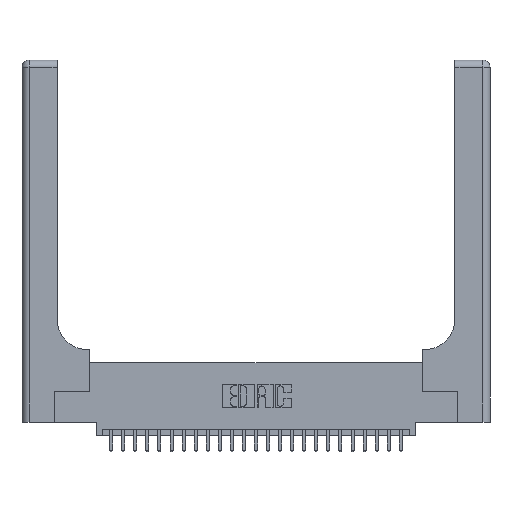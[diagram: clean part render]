
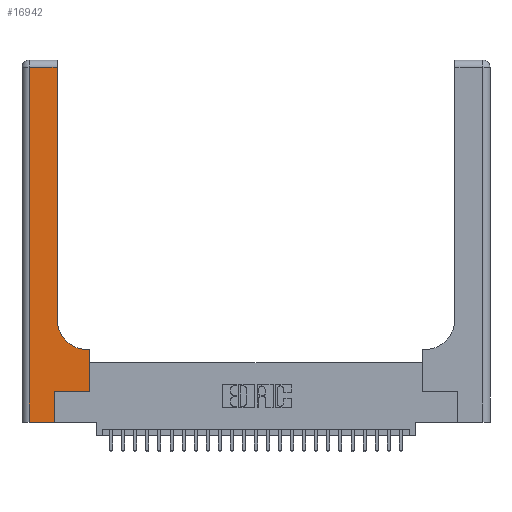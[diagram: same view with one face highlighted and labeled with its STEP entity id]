
A CAD part, top view. The second image highlights one B-rep face of the part: STEP entity #16942.
In plain terms, the highlighted planar face has unit normal (0, 0, 1).
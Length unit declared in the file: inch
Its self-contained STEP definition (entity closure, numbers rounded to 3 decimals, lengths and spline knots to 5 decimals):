
#304 = LINE ( 'NONE', #21245, #10974 ) ;
#325 = FACE_OUTER_BOUND ( 'NONE', #7812, .T. ) ;
#400 = DIRECTION ( 'NONE',  ( 1., 0., 0. ) ) ;
#538 = CARTESIAN_POINT ( 'NONE',  ( 0.269, 0., 0.37 ) ) ;
#1228 = VERTEX_POINT ( 'NONE', #18235 ) ;
#2016 = VECTOR ( 'NONE', #20267, 39.37008 ) ;
#2344 = DIRECTION ( 'NONE',  ( -1., 0., 0. ) ) ;
#2413 = LINE ( 'NONE', #10833, #7376 ) ;
#2420 = VERTEX_POINT ( 'NONE', #22962 ) ;
#2517 = CARTESIAN_POINT ( 'NONE',  ( 0.06, 0., 0.37 ) ) ;
#2800 = EDGE_CURVE ( 'NONE', #15787, #12456, #25503, .T. ) ;
#3006 = LINE ( 'NONE', #10348, #24642 ) ;
#4120 = VECTOR ( 'NONE', #6525, 39.37008 ) ;
#4416 = CARTESIAN_POINT ( 'NONE',  ( 0., 0., 0.37 ) ) ;
#4740 = VECTOR ( 'NONE', #14654, 39.37008 ) ;
#4775 = ORIENTED_EDGE ( 'NONE', *, *, #10673, .T. ) ;
#5481 = EDGE_CURVE ( 'NONE', #2420, #22334, #2413, .T. ) ;
#6018 = EDGE_CURVE ( 'NONE', #22334, #8219, #304, .T. ) ;
#6148 = CARTESIAN_POINT ( 'NONE',  ( 0., 3., 0.37 ) ) ;
#6196 = EDGE_CURVE ( 'NONE', #1228, #19878, #23060, .T. ) ;
#6348 = VECTOR ( 'NONE', #9417, 39.37008 ) ;
#6392 = CARTESIAN_POINT ( 'NONE',  ( 0.5585, 0.25, 0.37 ) ) ;
#6525 = DIRECTION ( 'NONE',  ( 1., 0., 0. ) ) ;
#7376 = VECTOR ( 'NONE', #2344, 39.37008 ) ;
#7528 = VECTOR ( 'NONE', #19000, 39.37008 ) ;
#7812 = EDGE_LOOP ( 'NONE', ( #13229, #25976, #10663, #18224, #12291, #20404, #9405, #4775, #8442 ) ) ;
#8219 = VERTEX_POINT ( 'NONE', #2517 ) ;
#8442 = ORIENTED_EDGE ( 'NONE', *, *, #2800, .T. ) ;
#8754 = EDGE_CURVE ( 'NONE', #12456, #2420, #22121, .T. ) ;
#9405 = ORIENTED_EDGE ( 'NONE', *, *, #25408, .T. ) ;
#9417 = DIRECTION ( 'NONE',  ( 1., 0., 0. ) ) ;
#9810 = CARTESIAN_POINT ( 'NONE',  ( 0.269, 0., 0.37 ) ) ;
#10348 = CARTESIAN_POINT ( 'NONE',  ( 0.2915, 0.6, 0.37 ) ) ;
#10452 = EDGE_CURVE ( 'NONE', #16365, #1228, #13914, .T. ) ;
#10465 = CARTESIAN_POINT ( 'NONE',  ( 0.5415, 0.6, 0.37 ) ) ;
#10531 = CARTESIAN_POINT ( 'NONE',  ( 0.2915, 3., 0.37 ) ) ;
#10663 = ORIENTED_EDGE ( 'NONE', *, *, #6018, .T. ) ;
#10673 = EDGE_CURVE ( 'NONE', #21796, #15787, #3006, .T. ) ;
#10833 = CARTESIAN_POINT ( 'NONE',  ( 0., 2.94, 0.37 ) ) ;
#10974 = VECTOR ( 'NONE', #23313, 39.37008 ) ;
#12291 = ORIENTED_EDGE ( 'NONE', *, *, #10452, .T. ) ;
#12456 = VERTEX_POINT ( 'NONE', #20928 ) ;
#12476 = DIRECTION ( 'NONE',  ( -1., 0., 0. ) ) ;
#12496 = DIRECTION ( 'NONE',  ( 0., 0., -1. ) ) ;
#13073 = CARTESIAN_POINT ( 'NONE',  ( 0.5585, 0.6, 0.37 ) ) ;
#13145 = DIRECTION ( 'NONE',  ( 0., 0., -1. ) ) ;
#13229 = ORIENTED_EDGE ( 'NONE', *, *, #8754, .T. ) ;
#13914 = LINE ( 'NONE', #9810, #2016 ) ;
#14654 = DIRECTION ( 'NONE',  ( 0., 1., 0. ) ) ;
#15787 = VERTEX_POINT ( 'NONE', #10465 ) ;
#16365 = VERTEX_POINT ( 'NONE', #538 ) ;
#16600 = CARTESIAN_POINT ( 'NONE',  ( 0.06, 2.94, 0.37 ) ) ;
#16914 = AXIS2_PLACEMENT_3D ( 'NONE', #25590, #13145, #400 ) ;
#16942 = ADVANCED_FACE ( 'NONE', ( #325 ), #24955, .F. ) ;
#18224 = ORIENTED_EDGE ( 'NONE', *, *, #21702, .T. ) ;
#18235 = CARTESIAN_POINT ( 'NONE',  ( 0.269, 0.25, 0.37 ) ) ;
#19000 = DIRECTION ( 'NONE',  ( 0., 1., 0. ) ) ;
#19878 = VERTEX_POINT ( 'NONE', #23185 ) ;
#20267 = DIRECTION ( 'NONE',  ( 0., 1., 0. ) ) ;
#20404 = ORIENTED_EDGE ( 'NONE', *, *, #6196, .T. ) ;
#20928 = CARTESIAN_POINT ( 'NONE',  ( 0.2915, 0.85, 0.37 ) ) ;
#21245 = CARTESIAN_POINT ( 'NONE',  ( 0.06, 3., 0.37 ) ) ;
#21413 = AXIS2_PLACEMENT_3D ( 'NONE', #6148, #12496, #27040 ) ;
#21702 = EDGE_CURVE ( 'NONE', #8219, #16365, #26995, .T. ) ;
#21796 = VERTEX_POINT ( 'NONE', #13073 ) ;
#22121 = LINE ( 'NONE', #10531, #4740 ) ;
#22334 = VERTEX_POINT ( 'NONE', #16600 ) ;
#22962 = CARTESIAN_POINT ( 'NONE',  ( 0.2915, 2.94, 0.37 ) ) ;
#23060 = LINE ( 'NONE', #26089, #6348 ) ;
#23185 = CARTESIAN_POINT ( 'NONE',  ( 0.5585, 0.25, 0.37 ) ) ;
#23313 = DIRECTION ( 'NONE',  ( 0., -1., 0. ) ) ;
#24193 = LINE ( 'NONE', #6392, #7528 ) ;
#24642 = VECTOR ( 'NONE', #12476, 39.37008 ) ;
#24955 = PLANE ( 'NONE',  #21413 ) ;
#25408 = EDGE_CURVE ( 'NONE', #19878, #21796, #24193, .T. ) ;
#25503 = CIRCLE ( 'NONE', #16914, 0.25 ) ;
#25590 = CARTESIAN_POINT ( 'NONE',  ( 0.5415, 0.85, 0.37 ) ) ;
#25976 = ORIENTED_EDGE ( 'NONE', *, *, #5481, .T. ) ;
#26089 = CARTESIAN_POINT ( 'NONE',  ( 0.269, 0.25, 0.37 ) ) ;
#26995 = LINE ( 'NONE', #4416, #4120 ) ;
#27040 = DIRECTION ( 'NONE',  ( -1., 0., 0. ) ) ;
